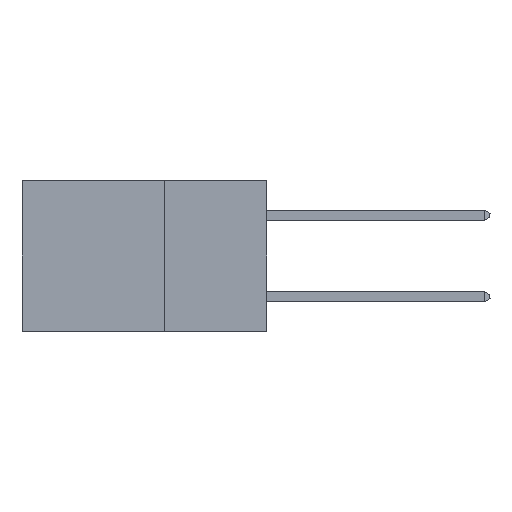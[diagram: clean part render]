
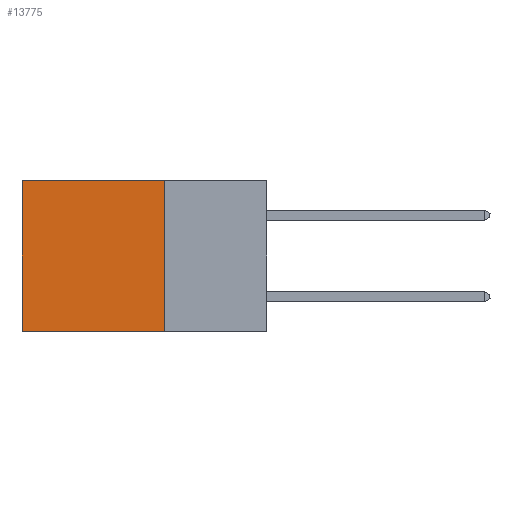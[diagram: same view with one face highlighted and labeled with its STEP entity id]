
A CAD part, left-side view. The second image highlights one B-rep face of the part: STEP entity #13775.
In plain terms, the highlighted planar face has unit normal (-1, 0, 0).
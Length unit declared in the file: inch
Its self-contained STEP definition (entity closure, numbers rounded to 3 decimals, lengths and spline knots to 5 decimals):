
#648 = VECTOR ( 'NONE', #10538, 39.37008 ) ;
#1263 = LINE ( 'NONE', #4741, #648 ) ;
#1383 = VERTEX_POINT ( 'NONE', #15484 ) ;
#1598 = VERTEX_POINT ( 'NONE', #6690 ) ;
#1969 = AXIS2_PLACEMENT_3D ( 'NONE', #17935, #23624, #12443 ) ;
#2549 = DIRECTION ( 'NONE',  ( 0., 1., 0. ) ) ;
#4741 = CARTESIAN_POINT ( 'NONE',  ( 0.2875, 0.25, 0. ) ) ;
#6554 = EDGE_CURVE ( 'NONE', #11507, #1598, #18832, .T. ) ;
#6614 = VECTOR ( 'NONE', #21636, 39.37008 ) ;
#6690 = CARTESIAN_POINT ( 'NONE',  ( 0.2875, 0.6, -0.37 ) ) ;
#6941 = ORIENTED_EDGE ( 'NONE', *, *, #16227, .T. ) ;
#8601 = PLANE ( 'NONE',  #1969 ) ;
#8742 = ORIENTED_EDGE ( 'NONE', *, *, #16157, .F. ) ;
#10071 = ORIENTED_EDGE ( 'NONE', *, *, #6554, .F. ) ;
#10362 = ORIENTED_EDGE ( 'NONE', *, *, #12666, .T. ) ;
#10538 = DIRECTION ( 'NONE',  ( 0., 1., 0. ) ) ;
#11507 = VERTEX_POINT ( 'NONE', #19774 ) ;
#12443 = DIRECTION ( 'NONE',  ( 0., 0., -1. ) ) ;
#12666 = EDGE_CURVE ( 'NONE', #16834, #1598, #23420, .T. ) ;
#12886 = VECTOR ( 'NONE', #14594, 39.37008 ) ;
#13424 = EDGE_LOOP ( 'NONE', ( #10362, #10071, #8742, #6941 ) ) ;
#13775 = ADVANCED_FACE ( 'NONE', ( #23525 ), #8601, .F. ) ;
#14401 = VECTOR ( 'NONE', #2549, 39.37008 ) ;
#14594 = DIRECTION ( 'NONE',  ( 0., 0., -1. ) ) ;
#15484 = CARTESIAN_POINT ( 'NONE',  ( 0.2875, 0.25, 0. ) ) ;
#16157 = EDGE_CURVE ( 'NONE', #1383, #11507, #21688, .T. ) ;
#16227 = EDGE_CURVE ( 'NONE', #1383, #16834, #1263, .T. ) ;
#16834 = VERTEX_POINT ( 'NONE', #21528 ) ;
#17935 = CARTESIAN_POINT ( 'NONE',  ( 0.2875, 0.25, 0. ) ) ;
#18832 = LINE ( 'NONE', #21437, #14401 ) ;
#19759 = CARTESIAN_POINT ( 'NONE',  ( 0.2875, 0.25, 0. ) ) ;
#19774 = CARTESIAN_POINT ( 'NONE',  ( 0.2875, 0.25, -0.37 ) ) ;
#21437 = CARTESIAN_POINT ( 'NONE',  ( 0.2875, 0.25, -0.37 ) ) ;
#21528 = CARTESIAN_POINT ( 'NONE',  ( 0.2875, 0.6, 0. ) ) ;
#21636 = DIRECTION ( 'NONE',  ( 0., 0., -1. ) ) ;
#21688 = LINE ( 'NONE', #19759, #6614 ) ;
#22188 = CARTESIAN_POINT ( 'NONE',  ( 0.2875, 0.6, 0. ) ) ;
#23420 = LINE ( 'NONE', #22188, #12886 ) ;
#23525 = FACE_OUTER_BOUND ( 'NONE', #13424, .T. ) ;
#23624 = DIRECTION ( 'NONE',  ( 1., 0., 0. ) ) ;
